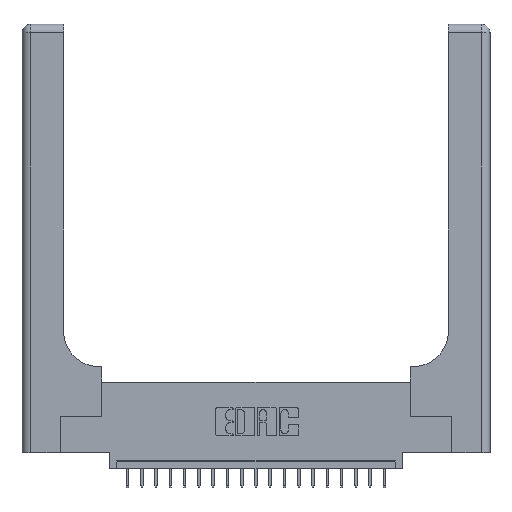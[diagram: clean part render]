
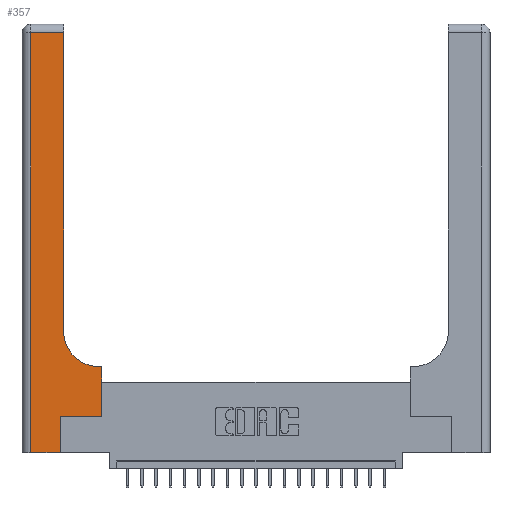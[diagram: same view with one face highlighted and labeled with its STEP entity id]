
A CAD part, top view. The second image highlights one B-rep face of the part: STEP entity #357.
In plain terms, the highlighted planar face has unit normal (0, 0, 1).
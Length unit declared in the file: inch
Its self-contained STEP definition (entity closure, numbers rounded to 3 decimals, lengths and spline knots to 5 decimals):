
#220 = EDGE_LOOP ( 'NONE', ( #16676, #20089, #21503, #11557, #22805, #10916, #1603, #6459, #6810 ) ) ;
#357 = ADVANCED_FACE ( 'NONE', ( #10619 ), #10848, .F. ) ;
#368 = CARTESIAN_POINT ( 'NONE',  ( 0.5585, 0.25, 0.37 ) ) ;
#904 = CARTESIAN_POINT ( 'NONE',  ( 0.06, 2.94, 0.37 ) ) ;
#1036 = VECTOR ( 'NONE', #1944, 39.37008 ) ;
#1198 = DIRECTION ( 'NONE',  ( 0., 0., -1. ) ) ;
#1213 = VERTEX_POINT ( 'NONE', #1395 ) ;
#1395 = CARTESIAN_POINT ( 'NONE',  ( 0.269, 0., 0.37 ) ) ;
#1603 = ORIENTED_EDGE ( 'NONE', *, *, #4579, .T. ) ;
#1944 = DIRECTION ( 'NONE',  ( 0., 1., 0. ) ) ;
#2561 = EDGE_CURVE ( 'NONE', #11382, #5456, #18089, .T. ) ;
#2682 = CARTESIAN_POINT ( 'NONE',  ( 0.5415, 0.85, 0.37 ) ) ;
#3710 = EDGE_CURVE ( 'NONE', #10906, #22420, #22598, .T. ) ;
#3808 = CARTESIAN_POINT ( 'NONE',  ( 0., 0., 0.37 ) ) ;
#4149 = CARTESIAN_POINT ( 'NONE',  ( 0.269, 0.25, 0.37 ) ) ;
#4579 = EDGE_CURVE ( 'NONE', #5456, #10906, #15676, .T. ) ;
#4699 = VECTOR ( 'NONE', #14077, 39.37008 ) ;
#5197 = LINE ( 'NONE', #3808, #21607 ) ;
#5456 = VERTEX_POINT ( 'NONE', #368 ) ;
#6187 = VECTOR ( 'NONE', #15382, 39.37008 ) ;
#6420 = CARTESIAN_POINT ( 'NONE',  ( 0.06, 0., 0.37 ) ) ;
#6459 = ORIENTED_EDGE ( 'NONE', *, *, #3710, .T. ) ;
#6487 = LINE ( 'NONE', #8123, #10406 ) ;
#6810 = ORIENTED_EDGE ( 'NONE', *, *, #19211, .T. ) ;
#6834 = VECTOR ( 'NONE', #15357, 39.37008 ) ;
#7806 = DIRECTION ( 'NONE',  ( -1., 0., 0. ) ) ;
#7809 = CARTESIAN_POINT ( 'NONE',  ( 0.2915, 3., 0.37 ) ) ;
#8123 = CARTESIAN_POINT ( 'NONE',  ( 0.269, 0., 0.37 ) ) ;
#8150 = DIRECTION ( 'NONE',  ( 1., 0., 0. ) ) ;
#8348 = CARTESIAN_POINT ( 'NONE',  ( 0.06, 3., 0.37 ) ) ;
#8397 = VERTEX_POINT ( 'NONE', #12366 ) ;
#8857 = EDGE_CURVE ( 'NONE', #8397, #9737, #12900, .T. ) ;
#9430 = DIRECTION ( 'NONE',  ( -1., 0., 0. ) ) ;
#9737 = VERTEX_POINT ( 'NONE', #904 ) ;
#10393 = DIRECTION ( 'NONE',  ( 0., 0., -1. ) ) ;
#10406 = VECTOR ( 'NONE', #20549, 39.37008 ) ;
#10619 = FACE_OUTER_BOUND ( 'NONE', #220, .T. ) ;
#10848 = PLANE ( 'NONE',  #22526 ) ;
#10874 = DIRECTION ( 'NONE',  ( 1., 0., 0. ) ) ;
#10906 = VERTEX_POINT ( 'NONE', #11042 ) ;
#10916 = ORIENTED_EDGE ( 'NONE', *, *, #2561, .T. ) ;
#11042 = CARTESIAN_POINT ( 'NONE',  ( 0.5585, 0.6, 0.37 ) ) ;
#11382 = VERTEX_POINT ( 'NONE', #20685 ) ;
#11557 = ORIENTED_EDGE ( 'NONE', *, *, #17445, .T. ) ;
#11881 = EDGE_CURVE ( 'NONE', #1213, #11382, #6487, .T. ) ;
#12366 = CARTESIAN_POINT ( 'NONE',  ( 0.2915, 2.94, 0.37 ) ) ;
#12900 = LINE ( 'NONE', #21646, #19534 ) ;
#14077 = DIRECTION ( 'NONE',  ( -1., 0., 0. ) ) ;
#15185 = VERTEX_POINT ( 'NONE', #6420 ) ;
#15215 = VECTOR ( 'NONE', #18192, 39.37008 ) ;
#15357 = DIRECTION ( 'NONE',  ( 0., -1., 0. ) ) ;
#15382 = DIRECTION ( 'NONE',  ( 0., 1., 0. ) ) ;
#15676 = LINE ( 'NONE', #22744, #1036 ) ;
#15753 = CARTESIAN_POINT ( 'NONE',  ( 0., 3., 0.37 ) ) ;
#16266 = EDGE_CURVE ( 'NONE', #9737, #15185, #17075, .T. ) ;
#16513 = LINE ( 'NONE', #7809, #6187 ) ;
#16676 = ORIENTED_EDGE ( 'NONE', *, *, #19193, .T. ) ;
#17075 = LINE ( 'NONE', #8348, #6834 ) ;
#17445 = EDGE_CURVE ( 'NONE', #15185, #1213, #5197, .T. ) ;
#18089 = LINE ( 'NONE', #4149, #15215 ) ;
#18192 = DIRECTION ( 'NONE',  ( 1., 0., 0. ) ) ;
#18297 = CARTESIAN_POINT ( 'NONE',  ( 0.5415, 0.6, 0.37 ) ) ;
#19059 = CIRCLE ( 'NONE', #22021, 0.25 ) ;
#19193 = EDGE_CURVE ( 'NONE', #19519, #8397, #16513, .T. ) ;
#19211 = EDGE_CURVE ( 'NONE', #22420, #19519, #19059, .T. ) ;
#19519 = VERTEX_POINT ( 'NONE', #20178 ) ;
#19534 = VECTOR ( 'NONE', #9430, 39.37008 ) ;
#20089 = ORIENTED_EDGE ( 'NONE', *, *, #8857, .T. ) ;
#20178 = CARTESIAN_POINT ( 'NONE',  ( 0.2915, 0.85, 0.37 ) ) ;
#20549 = DIRECTION ( 'NONE',  ( 0., 1., 0. ) ) ;
#20685 = CARTESIAN_POINT ( 'NONE',  ( 0.269, 0.25, 0.37 ) ) ;
#21308 = CARTESIAN_POINT ( 'NONE',  ( 0.2915, 0.6, 0.37 ) ) ;
#21503 = ORIENTED_EDGE ( 'NONE', *, *, #16266, .T. ) ;
#21607 = VECTOR ( 'NONE', #10874, 39.37008 ) ;
#21646 = CARTESIAN_POINT ( 'NONE',  ( 0., 2.94, 0.37 ) ) ;
#22021 = AXIS2_PLACEMENT_3D ( 'NONE', #2682, #1198, #8150 ) ;
#22420 = VERTEX_POINT ( 'NONE', #18297 ) ;
#22526 = AXIS2_PLACEMENT_3D ( 'NONE', #15753, #10393, #7806 ) ;
#22598 = LINE ( 'NONE', #21308, #4699 ) ;
#22744 = CARTESIAN_POINT ( 'NONE',  ( 0.5585, 0.25, 0.37 ) ) ;
#22805 = ORIENTED_EDGE ( 'NONE', *, *, #11881, .T. ) ;
